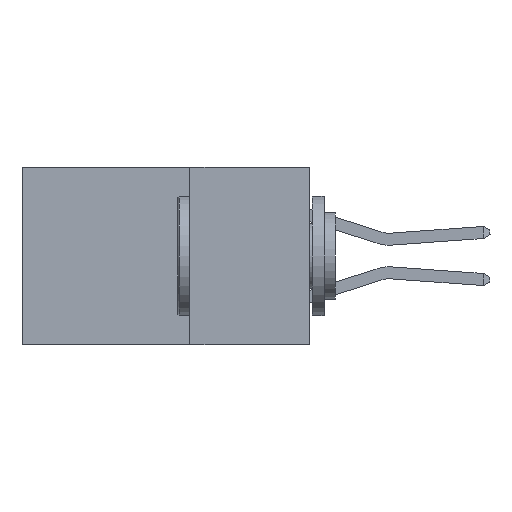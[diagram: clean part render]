
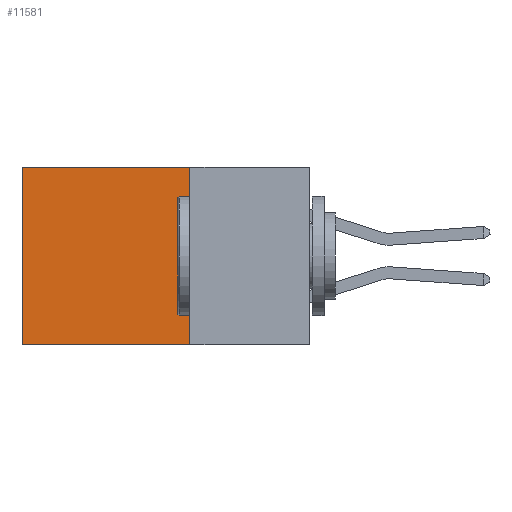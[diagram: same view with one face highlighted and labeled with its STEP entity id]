
A CAD part, left-side view. The second image highlights one B-rep face of the part: STEP entity #11581.
In plain terms, the highlighted planar face has unit normal (-1, 0, 0).
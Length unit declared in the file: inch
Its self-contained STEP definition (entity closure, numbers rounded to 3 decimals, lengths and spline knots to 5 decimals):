
#66 = CARTESIAN_POINT ( 'NONE',  ( 0.298, 0.6, -0.37 ) ) ;
#255 = ORIENTED_EDGE ( 'NONE', *, *, #15323, .T. ) ;
#467 = DIRECTION ( 'NONE',  ( 1., 0., 0. ) ) ;
#2162 = FACE_OUTER_BOUND ( 'NONE', #17972, .T. ) ;
#2820 = LINE ( 'NONE', #12969, #15708 ) ;
#5948 = VECTOR ( 'NONE', #19834, 39.37008 ) ;
#6275 = CARTESIAN_POINT ( 'NONE',  ( 0.298, 0.25, -0.37 ) ) ;
#6501 = LINE ( 'NONE', #9812, #5948 ) ;
#7453 = CARTESIAN_POINT ( 'NONE',  ( 0.298, 0.6, 0. ) ) ;
#7838 = LINE ( 'NONE', #6275, #20613 ) ;
#7955 = DIRECTION ( 'NONE',  ( 0., 1., 0. ) ) ;
#8529 = LINE ( 'NONE', #20531, #16920 ) ;
#9418 = EDGE_CURVE ( 'NONE', #16215, #10569, #2820, .T. ) ;
#9509 = AXIS2_PLACEMENT_3D ( 'NONE', #13854, #467, #12216 ) ;
#9632 = VERTEX_POINT ( 'NONE', #7453 ) ;
#9812 = CARTESIAN_POINT ( 'NONE',  ( 0.298, 0.6, 0. ) ) ;
#9828 = EDGE_CURVE ( 'NONE', #10569, #15188, #7838, .T. ) ;
#10555 = PLANE ( 'NONE',  #9509 ) ;
#10569 = VERTEX_POINT ( 'NONE', #14791 ) ;
#10580 = EDGE_CURVE ( 'NONE', #9632, #15188, #6501, .T. ) ;
#11261 = DIRECTION ( 'NONE',  ( 0., 0., -1. ) ) ;
#11581 = ADVANCED_FACE ( 'NONE', ( #2162 ), #10555, .F. ) ;
#12183 = DIRECTION ( 'NONE',  ( 0., 1., 0. ) ) ;
#12216 = DIRECTION ( 'NONE',  ( 0., 0., -1. ) ) ;
#12969 = CARTESIAN_POINT ( 'NONE',  ( 0.298, 0.25, 0. ) ) ;
#13854 = CARTESIAN_POINT ( 'NONE',  ( 0.298, 0.25, 0. ) ) ;
#14281 = ORIENTED_EDGE ( 'NONE', *, *, #9418, .F. ) ;
#14739 = CARTESIAN_POINT ( 'NONE',  ( 0.298, 0.25, 0. ) ) ;
#14791 = CARTESIAN_POINT ( 'NONE',  ( 0.298, 0.25, -0.37 ) ) ;
#15188 = VERTEX_POINT ( 'NONE', #66 ) ;
#15323 = EDGE_CURVE ( 'NONE', #16215, #9632, #8529, .T. ) ;
#15708 = VECTOR ( 'NONE', #11261, 39.37008 ) ;
#16215 = VERTEX_POINT ( 'NONE', #14739 ) ;
#16920 = VECTOR ( 'NONE', #12183, 39.37008 ) ;
#17972 = EDGE_LOOP ( 'NONE', ( #18595, #18029, #14281, #255 ) ) ;
#18029 = ORIENTED_EDGE ( 'NONE', *, *, #9828, .F. ) ;
#18595 = ORIENTED_EDGE ( 'NONE', *, *, #10580, .T. ) ;
#19834 = DIRECTION ( 'NONE',  ( 0., 0., -1. ) ) ;
#20531 = CARTESIAN_POINT ( 'NONE',  ( 0.298, 0.25, 0. ) ) ;
#20613 = VECTOR ( 'NONE', #7955, 39.37008 ) ;
